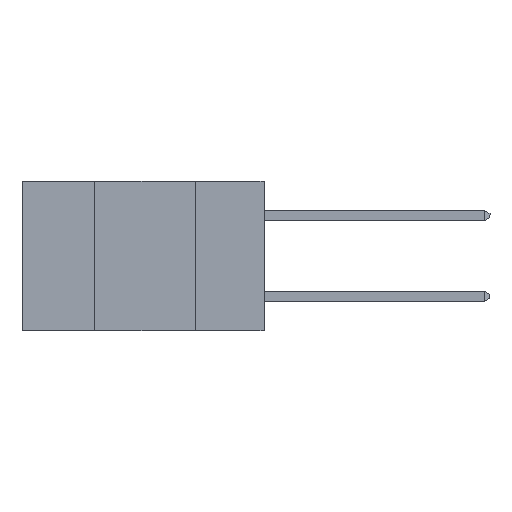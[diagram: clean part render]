
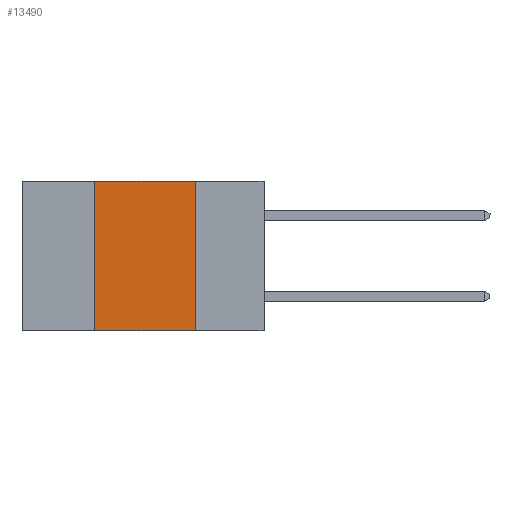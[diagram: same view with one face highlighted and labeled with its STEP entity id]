
A CAD part, left-side view. The second image highlights one B-rep face of the part: STEP entity #13490.
In plain terms, the highlighted planar face has unit normal (-1, 0, 0).
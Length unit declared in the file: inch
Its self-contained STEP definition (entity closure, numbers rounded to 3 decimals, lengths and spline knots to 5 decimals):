
#600 = EDGE_CURVE ( 'NONE', #3394, #6202, #10373, .T. ) ;
#812 = CARTESIAN_POINT ( 'NONE',  ( 0., 0.42, 0. ) ) ;
#876 = CARTESIAN_POINT ( 'NONE',  ( 0., 0.17, 0. ) ) ;
#998 = CARTESIAN_POINT ( 'NONE',  ( 0., 0.17, 0. ) ) ;
#1046 = VERTEX_POINT ( 'NONE', #6307 ) ;
#1205 = DIRECTION ( 'NONE',  ( 0., -1., 0. ) ) ;
#1516 = CARTESIAN_POINT ( 'NONE',  ( 0., 0.6, -0.37 ) ) ;
#1901 = CARTESIAN_POINT ( 'NONE',  ( 0., 0.17, -0.37 ) ) ;
#3080 = LINE ( 'NONE', #812, #8797 ) ;
#3394 = VERTEX_POINT ( 'NONE', #998 ) ;
#3489 = EDGE_LOOP ( 'NONE', ( #7125, #4217, #6424, #12995 ) ) ;
#4217 = ORIENTED_EDGE ( 'NONE', *, *, #8786, .F. ) ;
#4451 = VECTOR ( 'NONE', #10155, 39.37008 ) ;
#4698 = CARTESIAN_POINT ( 'NONE',  ( 0., 0.6, 0. ) ) ;
#4774 = EDGE_CURVE ( 'NONE', #1046, #11680, #3080, .T. ) ;
#5098 = FACE_OUTER_BOUND ( 'NONE', #3489, .T. ) ;
#5795 = DIRECTION ( 'NONE',  ( 0., -1., 0. ) ) ;
#6202 = VERTEX_POINT ( 'NONE', #1901 ) ;
#6307 = CARTESIAN_POINT ( 'NONE',  ( 0., 0.42, -0.37 ) ) ;
#6389 = DIRECTION ( 'NONE',  ( 1., 0., 0. ) ) ;
#6424 = ORIENTED_EDGE ( 'NONE', *, *, #4774, .F. ) ;
#7125 = ORIENTED_EDGE ( 'NONE', *, *, #600, .F. ) ;
#7169 = EDGE_CURVE ( 'NONE', #1046, #6202, #9238, .T. ) ;
#8227 = DIRECTION ( 'NONE',  ( 0., 0., 1. ) ) ;
#8650 = AXIS2_PLACEMENT_3D ( 'NONE', #12542, #6389, #13532 ) ;
#8786 = EDGE_CURVE ( 'NONE', #11680, #3394, #8846, .T. ) ;
#8797 = VECTOR ( 'NONE', #8227, 39.37008 ) ;
#8846 = LINE ( 'NONE', #4698, #13877 ) ;
#9238 = LINE ( 'NONE', #1516, #11623 ) ;
#10155 = DIRECTION ( 'NONE',  ( 0., 0., -1. ) ) ;
#10373 = LINE ( 'NONE', #876, #4451 ) ;
#10505 = PLANE ( 'NONE',  #8650 ) ;
#11623 = VECTOR ( 'NONE', #1205, 39.37008 ) ;
#11680 = VERTEX_POINT ( 'NONE', #13847 ) ;
#12542 = CARTESIAN_POINT ( 'NONE',  ( 0., 0.6, 0. ) ) ;
#12995 = ORIENTED_EDGE ( 'NONE', *, *, #7169, .T. ) ;
#13490 = ADVANCED_FACE ( 'NONE', ( #5098 ), #10505, .F. ) ;
#13532 = DIRECTION ( 'NONE',  ( 0., 0., -1. ) ) ;
#13847 = CARTESIAN_POINT ( 'NONE',  ( 0., 0.42, 0. ) ) ;
#13877 = VECTOR ( 'NONE', #5795, 39.37008 ) ;
